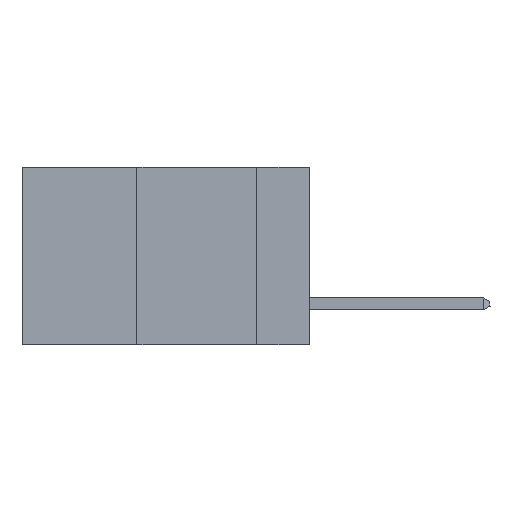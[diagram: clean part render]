
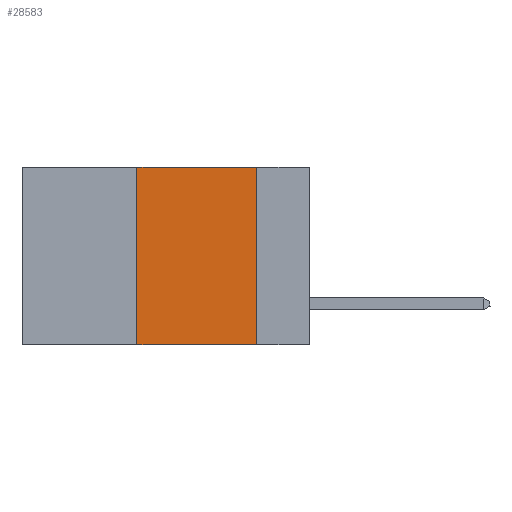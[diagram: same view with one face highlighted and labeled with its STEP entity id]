
A CAD part, left-side view. The second image highlights one B-rep face of the part: STEP entity #28583.
In plain terms, the highlighted planar face has unit normal (-1, 0, 0).
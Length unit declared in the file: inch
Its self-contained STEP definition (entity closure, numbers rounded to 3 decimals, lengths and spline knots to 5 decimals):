
#2351 = CARTESIAN_POINT ( 'NONE',  ( 0., 0.36, -0.37 ) ) ;
#3357 = LINE ( 'NONE', #45911, #14929 ) ;
#5717 = VECTOR ( 'NONE', #16301, 39.37008 ) ;
#6938 = EDGE_CURVE ( 'NONE', #34916, #15986, #11924, .T. ) ;
#7464 = ORIENTED_EDGE ( 'NONE', *, *, #25577, .F. ) ;
#9961 = CARTESIAN_POINT ( 'NONE',  ( 0., 0.6, 0. ) ) ;
#11061 = CARTESIAN_POINT ( 'NONE',  ( 0., 0.36, 0. ) ) ;
#11066 = AXIS2_PLACEMENT_3D ( 'NONE', #9961, #33008, #29249 ) ;
#11924 = LINE ( 'NONE', #16852, #14953 ) ;
#12802 = ORIENTED_EDGE ( 'NONE', *, *, #18185, .F. ) ;
#14818 = DIRECTION ( 'NONE',  ( 0., 0., -1. ) ) ;
#14929 = VECTOR ( 'NONE', #34144, 39.37008 ) ;
#14953 = VECTOR ( 'NONE', #28308, 39.37008 ) ;
#15986 = VERTEX_POINT ( 'NONE', #31209 ) ;
#16301 = DIRECTION ( 'NONE',  ( 0., -1., 0. ) ) ;
#16852 = CARTESIAN_POINT ( 'NONE',  ( 0., 0.6, 0. ) ) ;
#18185 = EDGE_CURVE ( 'NONE', #15986, #39650, #23659, .T. ) ;
#18758 = CARTESIAN_POINT ( 'NONE',  ( 0., 0.11, 0. ) ) ;
#18828 = ORIENTED_EDGE ( 'NONE', *, *, #48825, .T. ) ;
#23659 = LINE ( 'NONE', #18758, #46750 ) ;
#24400 = CARTESIAN_POINT ( 'NONE',  ( 0., 0.6, -0.37 ) ) ;
#25577 = EDGE_CURVE ( 'NONE', #26213, #34916, #3357, .T. ) ;
#26213 = VERTEX_POINT ( 'NONE', #2351 ) ;
#28308 = DIRECTION ( 'NONE',  ( 0., -1., 0. ) ) ;
#28583 = ADVANCED_FACE ( 'NONE', ( #30135 ), #41024, .F. ) ;
#28775 = LINE ( 'NONE', #24400, #5717 ) ;
#29249 = DIRECTION ( 'NONE',  ( 0., 0., -1. ) ) ;
#30135 = FACE_OUTER_BOUND ( 'NONE', #46367, .T. ) ;
#30677 = CARTESIAN_POINT ( 'NONE',  ( 0., 0.11, -0.37 ) ) ;
#31209 = CARTESIAN_POINT ( 'NONE',  ( 0., 0.11, 0. ) ) ;
#33008 = DIRECTION ( 'NONE',  ( 1., 0., 0. ) ) ;
#34144 = DIRECTION ( 'NONE',  ( 0., 0., 1. ) ) ;
#34916 = VERTEX_POINT ( 'NONE', #11061 ) ;
#39650 = VERTEX_POINT ( 'NONE', #30677 ) ;
#41024 = PLANE ( 'NONE',  #11066 ) ;
#43697 = ORIENTED_EDGE ( 'NONE', *, *, #6938, .F. ) ;
#45911 = CARTESIAN_POINT ( 'NONE',  ( 0., 0.36, 0. ) ) ;
#46367 = EDGE_LOOP ( 'NONE', ( #12802, #43697, #7464, #18828 ) ) ;
#46750 = VECTOR ( 'NONE', #14818, 39.37008 ) ;
#48825 = EDGE_CURVE ( 'NONE', #26213, #39650, #28775, .T. ) ;
